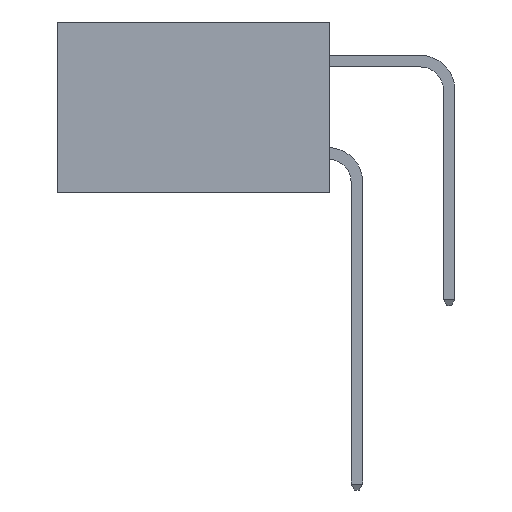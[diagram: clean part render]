
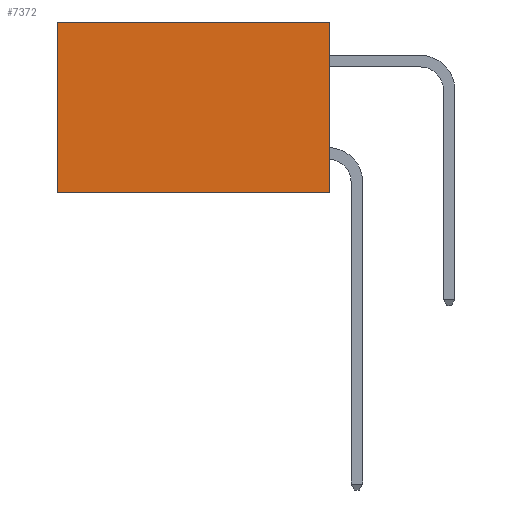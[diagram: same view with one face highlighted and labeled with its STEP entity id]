
A CAD part, left-side view. The second image highlights one B-rep face of the part: STEP entity #7372.
In plain terms, the highlighted planar face has unit normal (-1, 0, 0).
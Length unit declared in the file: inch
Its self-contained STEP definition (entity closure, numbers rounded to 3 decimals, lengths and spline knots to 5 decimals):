
#573 = DIRECTION ( 'NONE',  ( 0., 0., -1. ) ) ;
#1605 = ORIENTED_EDGE ( 'NONE', *, *, #19175, .T. ) ;
#1658 = CARTESIAN_POINT ( 'NONE',  ( 0.277, 0.59, -0.37 ) ) ;
#2867 = EDGE_CURVE ( 'NONE', #19463, #17347, #20816, .T. ) ;
#3286 = ORIENTED_EDGE ( 'NONE', *, *, #19744, .F. ) ;
#4160 = VERTEX_POINT ( 'NONE', #11719 ) ;
#4719 = CARTESIAN_POINT ( 'NONE',  ( 0.277, 0., -0.37 ) ) ;
#5866 = CARTESIAN_POINT ( 'NONE',  ( 0.277, 0., 0. ) ) ;
#6917 = DIRECTION ( 'NONE',  ( 0., 0., -1. ) ) ;
#7372 = ADVANCED_FACE ( 'NONE', ( #11700 ), #14225, .F. ) ;
#7573 = DIRECTION ( 'NONE',  ( 0., 1., 0. ) ) ;
#7576 = VECTOR ( 'NONE', #7573, 39.37008 ) ;
#7793 = CARTESIAN_POINT ( 'NONE',  ( 0.277, 0.59, -0.37 ) ) ;
#10765 = LINE ( 'NONE', #1658, #18594 ) ;
#11237 = ORIENTED_EDGE ( 'NONE', *, *, #2867, .F. ) ;
#11667 = EDGE_CURVE ( 'NONE', #19463, #4160, #16454, .T. ) ;
#11700 = FACE_OUTER_BOUND ( 'NONE', #19715, .T. ) ;
#11719 = CARTESIAN_POINT ( 'NONE',  ( 0.277, 0.59, 0. ) ) ;
#11747 = VERTEX_POINT ( 'NONE', #7793 ) ;
#12540 = VECTOR ( 'NONE', #18129, 39.37008 ) ;
#13580 = CARTESIAN_POINT ( 'NONE',  ( 0.277, 0., -0.37 ) ) ;
#14117 = DIRECTION ( 'NONE',  ( 0., 0., -1. ) ) ;
#14143 = DIRECTION ( 'NONE',  ( 1., 0., 0. ) ) ;
#14159 = CARTESIAN_POINT ( 'NONE',  ( 0.277, 0., -0.37 ) ) ;
#14225 = PLANE ( 'NONE',  #20023 ) ;
#16454 = LINE ( 'NONE', #17568, #7576 ) ;
#16850 = CARTESIAN_POINT ( 'NONE',  ( 0.277, 0., -0.37 ) ) ;
#16988 = LINE ( 'NONE', #4719, #12540 ) ;
#17347 = VERTEX_POINT ( 'NONE', #16850 ) ;
#17568 = CARTESIAN_POINT ( 'NONE',  ( 0.277, 0., 0. ) ) ;
#18029 = ORIENTED_EDGE ( 'NONE', *, *, #11667, .T. ) ;
#18129 = DIRECTION ( 'NONE',  ( 0., 1., 0. ) ) ;
#18594 = VECTOR ( 'NONE', #6917, 39.37008 ) ;
#19175 = EDGE_CURVE ( 'NONE', #4160, #11747, #10765, .T. ) ;
#19463 = VERTEX_POINT ( 'NONE', #5866 ) ;
#19715 = EDGE_LOOP ( 'NONE', ( #1605, #3286, #11237, #18029 ) ) ;
#19744 = EDGE_CURVE ( 'NONE', #17347, #11747, #16988, .T. ) ;
#20023 = AXIS2_PLACEMENT_3D ( 'NONE', #14159, #14143, #14117 ) ;
#20325 = VECTOR ( 'NONE', #573, 39.37008 ) ;
#20816 = LINE ( 'NONE', #13580, #20325 ) ;
